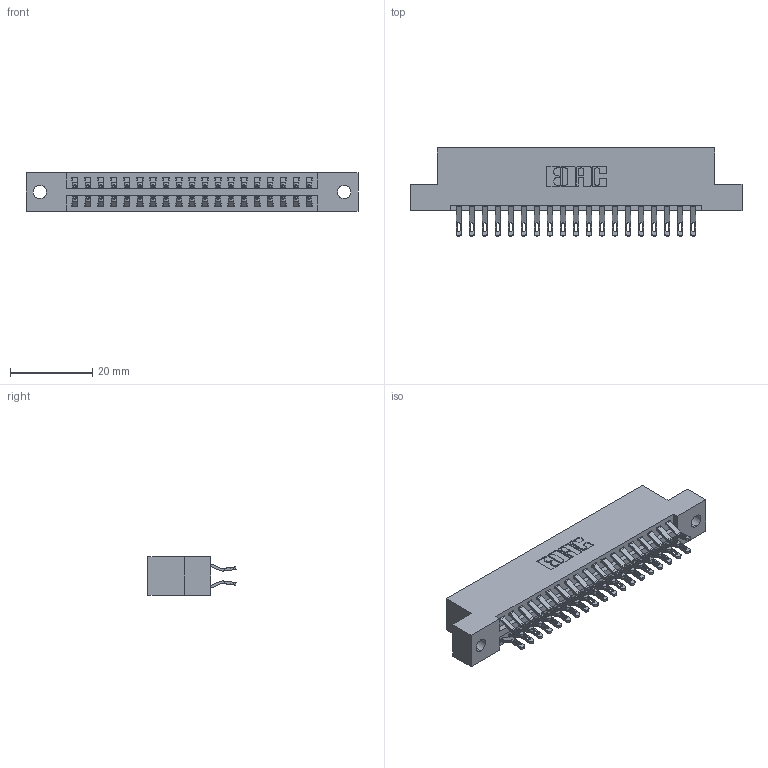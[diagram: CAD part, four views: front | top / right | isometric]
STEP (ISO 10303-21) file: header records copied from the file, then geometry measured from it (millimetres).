
FILE_DESCRIPTION (( 'STEP AP203' ), '1' );
FILE_NAME ('396-038-555-202.STEP', '2019-10-30T08:17:30', ( '' ), ( '' ), 'SwSTEP 2.0', 'SolidWorks 2016', '' );
FILE_SCHEMA (( 'CONFIG_CONTROL_DESIGN' ));
Length unit declared in the file: inch
Products named in the file (3): 346 Part_Flush Mounting Lugs - 0.128 Dia; 345-292-001_555 Tail; 396-038-555-202
Assembly tree (39 placements, depth 2):
  396-038-555-202
    346 Part_Flush Mounting Lugs - 0.128 Dia
    345-292-001_555 Tail  x38
Bounding box: 80.9 x 21.46 x 9.4 mm (x, y, z)
Volume: 7783.6 mm3; surface area: 10461.2 mm2
Topology: 39 solids, 39 shells, 2326 faces, 7283 edges, 4854 vertices
Faces by surface type: plane 1330, cylinder 996
Entity records: 15825 total; most frequent: CARTESIAN_POINT 2674, ORIENTED_EDGE 2578, DIRECTION 2377, EDGE_CURVE 1289, VECTOR 1061, LINE 1061, VERTEX_POINT 858, AXIS2_PLACEMENT_3D 658
